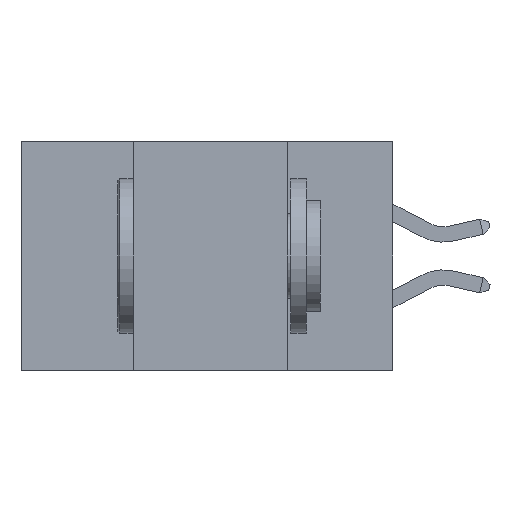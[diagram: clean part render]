
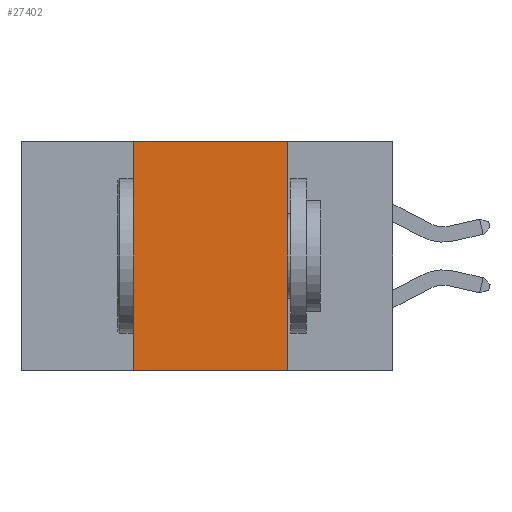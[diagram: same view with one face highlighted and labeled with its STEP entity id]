
A CAD part, left-side view. The second image highlights one B-rep face of the part: STEP entity #27402.
In plain terms, the highlighted planar face has unit normal (-1, 0, 0).
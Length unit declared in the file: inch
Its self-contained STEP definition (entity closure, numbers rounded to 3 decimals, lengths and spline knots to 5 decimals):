
#746 = EDGE_CURVE ( 'NONE', #3321, #8672, #33521, .T. ) ;
#842 = LINE ( 'NONE', #24459, #15427 ) ;
#2211 = ORIENTED_EDGE ( 'NONE', *, *, #25997, .F. ) ;
#3321 = VERTEX_POINT ( 'NONE', #26829 ) ;
#4274 = DIRECTION ( 'NONE',  ( 0., -1., 0. ) ) ;
#4386 = LINE ( 'NONE', #35865, #25585 ) ;
#4887 = AXIS2_PLACEMENT_3D ( 'NONE', #8083, #33808, #16765 ) ;
#4946 = CARTESIAN_POINT ( 'NONE',  ( 0., 0.17, -0.37 ) ) ;
#5661 = LINE ( 'NONE', #9929, #35237 ) ;
#7384 = DIRECTION ( 'NONE',  ( 0., 0., 1. ) ) ;
#8083 = CARTESIAN_POINT ( 'NONE',  ( 0., 0.6, 0. ) ) ;
#8191 = ORIENTED_EDGE ( 'NONE', *, *, #746, .F. ) ;
#8672 = VERTEX_POINT ( 'NONE', #27282 ) ;
#9929 = CARTESIAN_POINT ( 'NONE',  ( 0., 0.17, 0. ) ) ;
#10641 = EDGE_CURVE ( 'NONE', #8672, #16338, #5661, .T. ) ;
#11522 = EDGE_LOOP ( 'NONE', ( #30119, #8191, #2211, #17635 ) ) ;
#15128 = VERTEX_POINT ( 'NONE', #28800 ) ;
#15427 = VECTOR ( 'NONE', #4274, 39.37008 ) ;
#16338 = VERTEX_POINT ( 'NONE', #4946 ) ;
#16765 = DIRECTION ( 'NONE',  ( 0., 0., -1. ) ) ;
#16887 = EDGE_CURVE ( 'NONE', #15128, #16338, #842, .T. ) ;
#17635 = ORIENTED_EDGE ( 'NONE', *, *, #16887, .T. ) ;
#24459 = CARTESIAN_POINT ( 'NONE',  ( 0., 0.6, -0.37 ) ) ;
#25291 = PLANE ( 'NONE',  #4887 ) ;
#25585 = VECTOR ( 'NONE', #7384, 39.37008 ) ;
#25997 = EDGE_CURVE ( 'NONE', #15128, #3321, #4386, .T. ) ;
#26645 = CARTESIAN_POINT ( 'NONE',  ( 0., 0.6, 0. ) ) ;
#26766 = DIRECTION ( 'NONE',  ( 0., -1., 0. ) ) ;
#26829 = CARTESIAN_POINT ( 'NONE',  ( 0., 0.42, 0. ) ) ;
#27282 = CARTESIAN_POINT ( 'NONE',  ( 0., 0.17, 0. ) ) ;
#27402 = ADVANCED_FACE ( 'NONE', ( #31221 ), #25291, .F. ) ;
#28800 = CARTESIAN_POINT ( 'NONE',  ( 0., 0.42, -0.37 ) ) ;
#30119 = ORIENTED_EDGE ( 'NONE', *, *, #10641, .F. ) ;
#31221 = FACE_OUTER_BOUND ( 'NONE', #11522, .T. ) ;
#33521 = LINE ( 'NONE', #26645, #35286 ) ;
#33808 = DIRECTION ( 'NONE',  ( 1., 0., 0. ) ) ;
#35237 = VECTOR ( 'NONE', #35578, 39.37008 ) ;
#35286 = VECTOR ( 'NONE', #26766, 39.37008 ) ;
#35578 = DIRECTION ( 'NONE',  ( 0., 0., -1. ) ) ;
#35865 = CARTESIAN_POINT ( 'NONE',  ( 0., 0.42, 0. ) ) ;
